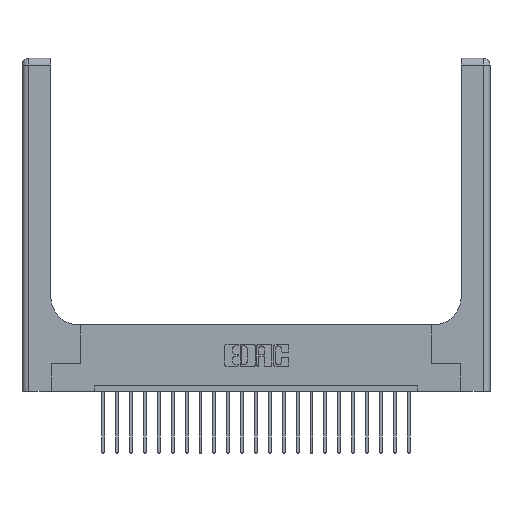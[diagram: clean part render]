
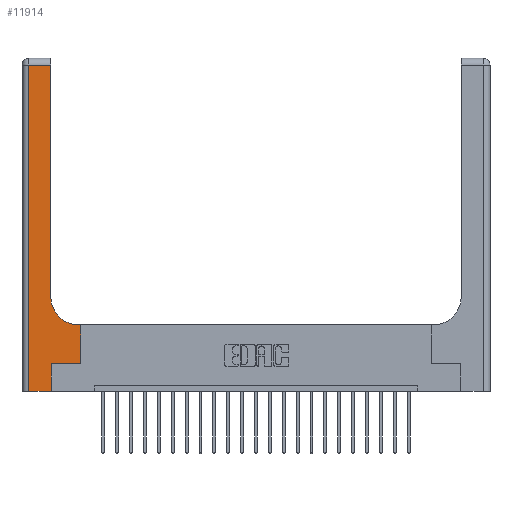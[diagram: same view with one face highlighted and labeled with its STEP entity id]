
A CAD part, top view. The second image highlights one B-rep face of the part: STEP entity #11914.
In plain terms, the highlighted planar face has unit normal (0, 0, 1).
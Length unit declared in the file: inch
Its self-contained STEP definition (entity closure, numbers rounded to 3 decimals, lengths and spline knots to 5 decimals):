
#397 = LINE ( 'NONE', #7704, #11254 ) ;
#408 = ORIENTED_EDGE ( 'NONE', *, *, #645, .T. ) ;
#600 = CARTESIAN_POINT ( 'NONE',  ( 0.26, 2.94, 0.37 ) ) ;
#645 = EDGE_CURVE ( 'NONE', #1830, #870, #397, .T. ) ;
#870 = VERTEX_POINT ( 'NONE', #3173 ) ;
#876 = DIRECTION ( 'NONE',  ( 0., -1., 0. ) ) ;
#1027 = CARTESIAN_POINT ( 'NONE',  ( 0.06, 3., 0.37 ) ) ;
#1042 = LINE ( 'NONE', #19827, #14078 ) ;
#1051 = ORIENTED_EDGE ( 'NONE', *, *, #4687, .T. ) ;
#1830 = VERTEX_POINT ( 'NONE', #600 ) ;
#1870 = AXIS2_PLACEMENT_3D ( 'NONE', #6753, #3283, #6831 ) ;
#2001 = LINE ( 'NONE', #4588, #2265 ) ;
#2265 = VECTOR ( 'NONE', #13425, 39.37008 ) ;
#2416 = ORIENTED_EDGE ( 'NONE', *, *, #15933, .T. ) ;
#2494 = DIRECTION ( 'NONE',  ( -1., 0., 0. ) ) ;
#2502 = CARTESIAN_POINT ( 'NONE',  ( 0.265, 0.25, 0.37 ) ) ;
#2999 = DIRECTION ( 'NONE',  ( 1., 0., 0. ) ) ;
#3071 = CARTESIAN_POINT ( 'NONE',  ( 0., 0., 0.37 ) ) ;
#3168 = CARTESIAN_POINT ( 'NONE',  ( 0.528, 0.6, 0.37 ) ) ;
#3173 = CARTESIAN_POINT ( 'NONE',  ( 0.06, 2.94, 0.37 ) ) ;
#3283 = DIRECTION ( 'NONE',  ( 0., 0., -1. ) ) ;
#3430 = VERTEX_POINT ( 'NONE', #12399 ) ;
#3848 = VERTEX_POINT ( 'NONE', #3168 ) ;
#3973 = ORIENTED_EDGE ( 'NONE', *, *, #20391, .T. ) ;
#4075 = EDGE_CURVE ( 'NONE', #5024, #4227, #7192, .T. ) ;
#4097 = CARTESIAN_POINT ( 'NONE',  ( 0.51, 0.6, 0.37 ) ) ;
#4227 = VERTEX_POINT ( 'NONE', #4995 ) ;
#4588 = CARTESIAN_POINT ( 'NONE',  ( 0.26, 0.6, 0.37 ) ) ;
#4687 = EDGE_CURVE ( 'NONE', #4814, #1830, #1042, .T. ) ;
#4814 = VERTEX_POINT ( 'NONE', #9720 ) ;
#4995 = CARTESIAN_POINT ( 'NONE',  ( 0.265, 0., 0.37 ) ) ;
#5024 = VERTEX_POINT ( 'NONE', #15295 ) ;
#5242 = FACE_OUTER_BOUND ( 'NONE', #15171, .T. ) ;
#6753 = CARTESIAN_POINT ( 'NONE',  ( 0., 3., 0.37 ) ) ;
#6831 = DIRECTION ( 'NONE',  ( -1., 0., 0. ) ) ;
#7192 = LINE ( 'NONE', #3071, #15707 ) ;
#7286 = CARTESIAN_POINT ( 'NONE',  ( 0.51, 0.85, 0.37 ) ) ;
#7310 = EDGE_CURVE ( 'NONE', #870, #5024, #15820, .T. ) ;
#7464 = EDGE_CURVE ( 'NONE', #3848, #15730, #2001, .T. ) ;
#7527 = AXIS2_PLACEMENT_3D ( 'NONE', #7286, #8845, #13892 ) ;
#7635 = LINE ( 'NONE', #2502, #16946 ) ;
#7704 = CARTESIAN_POINT ( 'NONE',  ( 0., 2.94, 0.37 ) ) ;
#8055 = ORIENTED_EDGE ( 'NONE', *, *, #7464, .T. ) ;
#8845 = DIRECTION ( 'NONE',  ( 0., 0., -1. ) ) ;
#9271 = DIRECTION ( 'NONE',  ( 1., 0., 0. ) ) ;
#9720 = CARTESIAN_POINT ( 'NONE',  ( 0.26, 0.85, 0.37 ) ) ;
#9778 = EDGE_CURVE ( 'NONE', #3430, #3848, #11172, .T. ) ;
#11172 = LINE ( 'NONE', #20919, #12518 ) ;
#11254 = VECTOR ( 'NONE', #2494, 39.37008 ) ;
#11619 = CIRCLE ( 'NONE', #7527, 0.25 ) ;
#11914 = ADVANCED_FACE ( 'NONE', ( #5242 ), #15025, .F. ) ;
#12399 = CARTESIAN_POINT ( 'NONE',  ( 0.528, 0.25, 0.37 ) ) ;
#12518 = VECTOR ( 'NONE', #21132, 39.37008 ) ;
#13425 = DIRECTION ( 'NONE',  ( -1., 0., 0. ) ) ;
#13892 = DIRECTION ( 'NONE',  ( 1., 0., 0. ) ) ;
#14078 = VECTOR ( 'NONE', #19528, 39.37008 ) ;
#14932 = ORIENTED_EDGE ( 'NONE', *, *, #4075, .T. ) ;
#15025 = PLANE ( 'NONE',  #1870 ) ;
#15084 = DIRECTION ( 'NONE',  ( 0., 1., 0. ) ) ;
#15171 = EDGE_LOOP ( 'NONE', ( #1051, #408, #20425, #14932, #2416, #3973, #15229, #8055, #15640 ) ) ;
#15229 = ORIENTED_EDGE ( 'NONE', *, *, #9778, .T. ) ;
#15289 = VECTOR ( 'NONE', #876, 39.37008 ) ;
#15295 = CARTESIAN_POINT ( 'NONE',  ( 0.06, 0., 0.37 ) ) ;
#15536 = CARTESIAN_POINT ( 'NONE',  ( 0.265, 0.25, 0.37 ) ) ;
#15640 = ORIENTED_EDGE ( 'NONE', *, *, #20292, .T. ) ;
#15707 = VECTOR ( 'NONE', #2999, 39.37008 ) ;
#15730 = VERTEX_POINT ( 'NONE', #4097 ) ;
#15820 = LINE ( 'NONE', #1027, #15289 ) ;
#15933 = EDGE_CURVE ( 'NONE', #4227, #20094, #19803, .T. ) ;
#16946 = VECTOR ( 'NONE', #9271, 39.37008 ) ;
#18560 = CARTESIAN_POINT ( 'NONE',  ( 0.265, 0., 0.37 ) ) ;
#19528 = DIRECTION ( 'NONE',  ( 0., 1., 0. ) ) ;
#19803 = LINE ( 'NONE', #18560, #20354 ) ;
#19827 = CARTESIAN_POINT ( 'NONE',  ( 0.26, 3., 0.37 ) ) ;
#20094 = VERTEX_POINT ( 'NONE', #15536 ) ;
#20292 = EDGE_CURVE ( 'NONE', #15730, #4814, #11619, .T. ) ;
#20354 = VECTOR ( 'NONE', #15084, 39.37008 ) ;
#20391 = EDGE_CURVE ( 'NONE', #20094, #3430, #7635, .T. ) ;
#20425 = ORIENTED_EDGE ( 'NONE', *, *, #7310, .T. ) ;
#20919 = CARTESIAN_POINT ( 'NONE',  ( 0.528, 0.25, 0.37 ) ) ;
#21132 = DIRECTION ( 'NONE',  ( 0., 1., 0. ) ) ;
